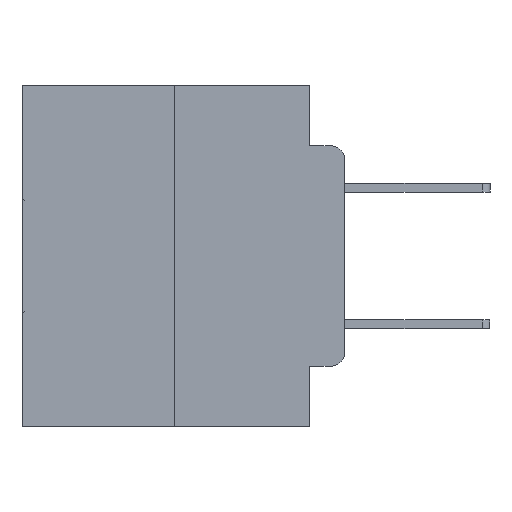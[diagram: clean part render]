
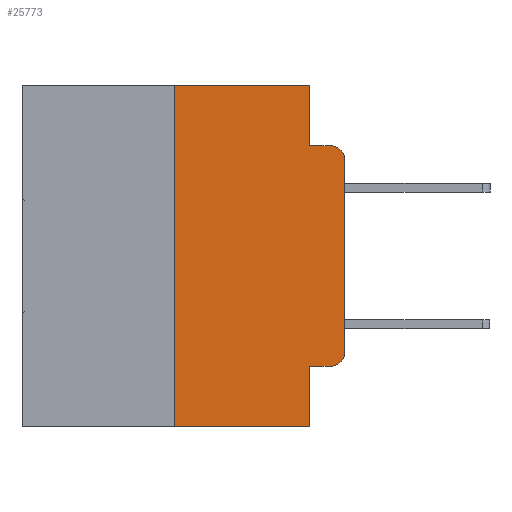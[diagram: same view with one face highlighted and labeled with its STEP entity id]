
A CAD part, left-side view. The second image highlights one B-rep face of the part: STEP entity #25773.
In plain terms, the highlighted planar face has unit normal (-1, 0, 0).
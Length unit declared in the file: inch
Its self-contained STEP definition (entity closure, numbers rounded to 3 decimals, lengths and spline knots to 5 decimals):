
#6 = VERTEX_POINT ( 'NONE', #11611 ) ;
#515 = VERTEX_POINT ( 'NONE', #11109 ) ;
#764 = EDGE_CURVE ( 'NONE', #15492, #2473, #12189, .T. ) ;
#1203 = EDGE_CURVE ( 'NONE', #23016, #1419, #12171, .T. ) ;
#1226 = VECTOR ( 'NONE', #21180, 39.37008 ) ;
#1419 = VERTEX_POINT ( 'NONE', #14608 ) ;
#1854 = ORIENTED_EDGE ( 'NONE', *, *, #19274, .F. ) ;
#1990 = VERTEX_POINT ( 'NONE', #27463 ) ;
#2221 = DIRECTION ( 'NONE',  ( 0., -1., 0. ) ) ;
#2473 = VERTEX_POINT ( 'NONE', #24121 ) ;
#3159 = LINE ( 'NONE', #12384, #14362 ) ;
#3602 = ORIENTED_EDGE ( 'NONE', *, *, #764, .T. ) ;
#3866 = ORIENTED_EDGE ( 'NONE', *, *, #1203, .F. ) ;
#4496 = DIRECTION ( 'NONE',  ( 0., 0., -1. ) ) ;
#4562 = AXIS2_PLACEMENT_3D ( 'NONE', #7728, #19038, #22651 ) ;
#4834 = LINE ( 'NONE', #26392, #15967 ) ;
#6076 = VECTOR ( 'NONE', #27476, 39.37008 ) ;
#6155 = ORIENTED_EDGE ( 'NONE', *, *, #14905, .T. ) ;
#6294 = AXIS2_PLACEMENT_3D ( 'NONE', #12716, #21565, #8418 ) ;
#6643 = VECTOR ( 'NONE', #19903, 39.37008 ) ;
#6797 = DIRECTION ( 'NONE',  ( -1., 0., 0. ) ) ;
#7174 = ORIENTED_EDGE ( 'NONE', *, *, #20718, .F. ) ;
#7331 = CARTESIAN_POINT ( 'NONE',  ( 0., 0.25, -0.5 ) ) ;
#7348 = LINE ( 'NONE', #15528, #6643 ) ;
#7440 = CARTESIAN_POINT ( 'NONE',  ( 0., 0.473, 0. ) ) ;
#7728 = CARTESIAN_POINT ( 'NONE',  ( 0., 0.02, -0.1085 ) ) ;
#8418 = DIRECTION ( 'NONE',  ( 0., 0., -1. ) ) ;
#9825 = ORIENTED_EDGE ( 'NONE', *, *, #15804, .T. ) ;
#10360 = DIRECTION ( 'NONE',  ( 0., 0., 1. ) ) ;
#11109 = CARTESIAN_POINT ( 'NONE',  ( 0., 0.051, -0.5 ) ) ;
#11611 = CARTESIAN_POINT ( 'NONE',  ( 0., 0.02, -0.4115 ) ) ;
#11728 = DIRECTION ( 'NONE',  ( 0., -1., 0. ) ) ;
#11913 = CARTESIAN_POINT ( 'NONE',  ( 0., 0.051, -0.0885 ) ) ;
#12171 = LINE ( 'NONE', #7440, #17311 ) ;
#12189 = CIRCLE ( 'NONE', #4562, 0.02 ) ;
#12384 = CARTESIAN_POINT ( 'NONE',  ( 0., 0.25, 0. ) ) ;
#12393 = ORIENTED_EDGE ( 'NONE', *, *, #22139, .F. ) ;
#12716 = CARTESIAN_POINT ( 'NONE',  ( 0., 0.473, 0. ) ) ;
#13205 = ORIENTED_EDGE ( 'NONE', *, *, #27804, .F. ) ;
#13300 = VECTOR ( 'NONE', #2221, 39.37008 ) ;
#13372 = VECTOR ( 'NONE', #11728, 39.37008 ) ;
#13441 = EDGE_CURVE ( 'NONE', #6, #16200, #16395, .T. ) ;
#14362 = VECTOR ( 'NONE', #10360, 39.37008 ) ;
#14608 = CARTESIAN_POINT ( 'NONE',  ( 0., 0.051, 0. ) ) ;
#14615 = LINE ( 'NONE', #17016, #1226 ) ;
#14905 = EDGE_CURVE ( 'NONE', #1990, #6, #19762, .T. ) ;
#15492 = VERTEX_POINT ( 'NONE', #24360 ) ;
#15528 = CARTESIAN_POINT ( 'NONE',  ( 0., 0.473, -0.5 ) ) ;
#15804 = EDGE_CURVE ( 'NONE', #16200, #15492, #14615, .T. ) ;
#15967 = VECTOR ( 'NONE', #4496, 39.37008 ) ;
#16131 = CARTESIAN_POINT ( 'NONE',  ( 0., 0., -0.3915 ) ) ;
#16200 = VERTEX_POINT ( 'NONE', #16131 ) ;
#16395 = CIRCLE ( 'NONE', #18114, 0.02 ) ;
#17016 = CARTESIAN_POINT ( 'NONE',  ( 0., 0., 0. ) ) ;
#17297 = DIRECTION ( 'NONE',  ( 0., -1., 0. ) ) ;
#17311 = VECTOR ( 'NONE', #17297, 39.37008 ) ;
#17792 = VERTEX_POINT ( 'NONE', #7331 ) ;
#17875 = EDGE_LOOP ( 'NONE', ( #9825, #3602, #13205, #12393, #3866, #7174, #24177, #1854, #6155, #25491 ) ) ;
#18114 = AXIS2_PLACEMENT_3D ( 'NONE', #20005, #6797, #22148 ) ;
#18255 = CARTESIAN_POINT ( 'NONE',  ( 0., 0.051, -0.0885 ) ) ;
#19038 = DIRECTION ( 'NONE',  ( -1., 0., 0. ) ) ;
#19163 = LINE ( 'NONE', #18255, #13372 ) ;
#19274 = EDGE_CURVE ( 'NONE', #1990, #515, #23561, .T. ) ;
#19394 = PLANE ( 'NONE',  #6294 ) ;
#19762 = LINE ( 'NONE', #28430, #13300 ) ;
#19774 = VERTEX_POINT ( 'NONE', #11913 ) ;
#19903 = DIRECTION ( 'NONE',  ( 0., -1., 0. ) ) ;
#20005 = CARTESIAN_POINT ( 'NONE',  ( 0., 0.02, -0.3915 ) ) ;
#20718 = EDGE_CURVE ( 'NONE', #17792, #23016, #3159, .T. ) ;
#21180 = DIRECTION ( 'NONE',  ( 0., 0., 1. ) ) ;
#21457 = EDGE_CURVE ( 'NONE', #17792, #515, #7348, .T. ) ;
#21565 = DIRECTION ( 'NONE',  ( 1., 0., 0. ) ) ;
#22139 = EDGE_CURVE ( 'NONE', #1419, #19774, #4834, .T. ) ;
#22148 = DIRECTION ( 'NONE',  ( 0., 0., -1. ) ) ;
#22651 = DIRECTION ( 'NONE',  ( 0., 0., -1. ) ) ;
#22963 = FACE_OUTER_BOUND ( 'NONE', #17875, .T. ) ;
#23016 = VERTEX_POINT ( 'NONE', #23921 ) ;
#23561 = LINE ( 'NONE', #25381, #6076 ) ;
#23921 = CARTESIAN_POINT ( 'NONE',  ( 0., 0.25, 0. ) ) ;
#24121 = CARTESIAN_POINT ( 'NONE',  ( 0., 0.02, -0.0885 ) ) ;
#24177 = ORIENTED_EDGE ( 'NONE', *, *, #21457, .T. ) ;
#24360 = CARTESIAN_POINT ( 'NONE',  ( 0., 0., -0.1085 ) ) ;
#25381 = CARTESIAN_POINT ( 'NONE',  ( 0., 0.051, 0. ) ) ;
#25491 = ORIENTED_EDGE ( 'NONE', *, *, #13441, .T. ) ;
#25773 = ADVANCED_FACE ( 'NONE', ( #22963 ), #19394, .F. ) ;
#26392 = CARTESIAN_POINT ( 'NONE',  ( 0., 0.051, 0. ) ) ;
#27463 = CARTESIAN_POINT ( 'NONE',  ( 0., 0.051, -0.4115 ) ) ;
#27476 = DIRECTION ( 'NONE',  ( 0., 0., -1. ) ) ;
#27804 = EDGE_CURVE ( 'NONE', #19774, #2473, #19163, .T. ) ;
#28430 = CARTESIAN_POINT ( 'NONE',  ( 0., 0.051, -0.4115 ) ) ;
